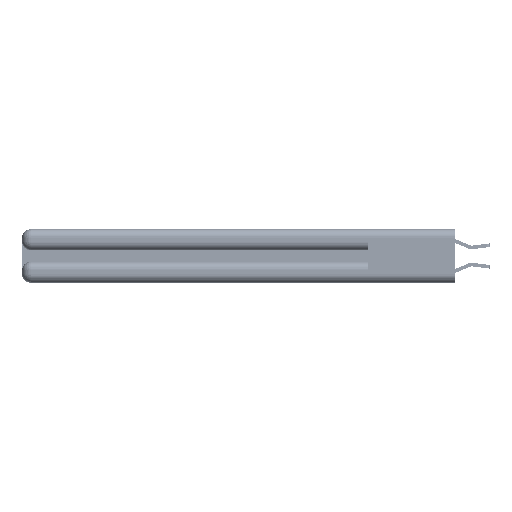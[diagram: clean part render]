
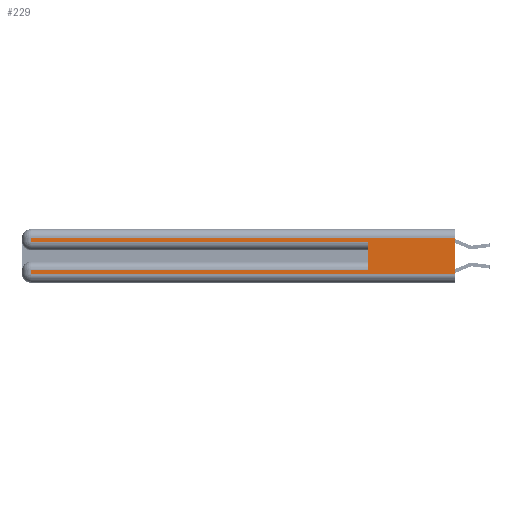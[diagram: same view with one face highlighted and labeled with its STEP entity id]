
A CAD part, left-side view. The second image highlights one B-rep face of the part: STEP entity #229.
In plain terms, the highlighted planar face has unit normal (-1, 0, 0).
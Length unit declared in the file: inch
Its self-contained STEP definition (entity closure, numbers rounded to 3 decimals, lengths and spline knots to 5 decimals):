
#146 = DIRECTION ( 'NONE',  ( 0., 0., -1. ) ) ;
#229 = ADVANCED_FACE ( 'NONE', ( #24275 ), #35878, .F. ) ;
#1392 = CARTESIAN_POINT ( 'NONE',  ( 0., 2.94, 0.31 ) ) ;
#1485 = DIRECTION ( 'NONE',  ( 0., 0., -1. ) ) ;
#1652 = LINE ( 'NONE', #9821, #9694 ) ;
#2906 = DIRECTION ( 'NONE',  ( 0., 0., 1. ) ) ;
#3354 = ORIENTED_EDGE ( 'NONE', *, *, #12501, .T. ) ;
#3734 = LINE ( 'NONE', #18161, #14110 ) ;
#4711 = VERTEX_POINT ( 'NONE', #18787 ) ;
#4900 = VERTEX_POINT ( 'NONE', #19917 ) ;
#5109 = DIRECTION ( 'NONE',  ( 0., 1., 0. ) ) ;
#6617 = VERTEX_POINT ( 'NONE', #23545 ) ;
#6716 = ORIENTED_EDGE ( 'NONE', *, *, #29918, .T. ) ;
#6874 = CARTESIAN_POINT ( 'NONE',  ( 0., 2.94, 0.285 ) ) ;
#9539 = VECTOR ( 'NONE', #30408, 39.37008 ) ;
#9694 = VECTOR ( 'NONE', #26918, 39.37008 ) ;
#9821 = CARTESIAN_POINT ( 'NONE',  ( 0., 0., 0.06 ) ) ;
#9845 = CARTESIAN_POINT ( 'NONE',  ( 0., 0., 0.37 ) ) ;
#9927 = VECTOR ( 'NONE', #5109, 39.37008 ) ;
#10403 = VECTOR ( 'NONE', #15825, 39.37008 ) ;
#11476 = EDGE_LOOP ( 'NONE', ( #21089, #34131, #6716, #29135, #17779, #20069, #21492, #3354 ) ) ;
#11734 = VERTEX_POINT ( 'NONE', #6874 ) ;
#12501 = EDGE_CURVE ( 'NONE', #4900, #4711, #1652, .T. ) ;
#14110 = VECTOR ( 'NONE', #146, 39.37008 ) ;
#14244 = VECTOR ( 'NONE', #37035, 39.37008 ) ;
#15766 = VERTEX_POINT ( 'NONE', #30734 ) ;
#15825 = DIRECTION ( 'NONE',  ( 0., 1., 0. ) ) ;
#16024 = VECTOR ( 'NONE', #2906, 39.37008 ) ;
#16754 = VERTEX_POINT ( 'NONE', #34576 ) ;
#17735 = CARTESIAN_POINT ( 'NONE',  ( 0., 0., 0.285 ) ) ;
#17779 = ORIENTED_EDGE ( 'NONE', *, *, #35022, .F. ) ;
#18161 = CARTESIAN_POINT ( 'NONE',  ( 0., 0., 0.37 ) ) ;
#18787 = CARTESIAN_POINT ( 'NONE',  ( 0., 0., 0.06 ) ) ;
#18814 = CARTESIAN_POINT ( 'NONE',  ( 0., 2.94, 0.37 ) ) ;
#19149 = LINE ( 'NONE', #19717, #9927 ) ;
#19717 = CARTESIAN_POINT ( 'NONE',  ( 0., 0., 0.085 ) ) ;
#19744 = EDGE_CURVE ( 'NONE', #16754, #31587, #21523, .T. ) ;
#19830 = LINE ( 'NONE', #17735, #30695 ) ;
#19917 = CARTESIAN_POINT ( 'NONE',  ( 0., 2.94, 0.06 ) ) ;
#20069 = ORIENTED_EDGE ( 'NONE', *, *, #35955, .T. ) ;
#21089 = ORIENTED_EDGE ( 'NONE', *, *, #23255, .F. ) ;
#21492 = ORIENTED_EDGE ( 'NONE', *, *, #27458, .T. ) ;
#21523 = LINE ( 'NONE', #29721, #10403 ) ;
#22397 = LINE ( 'NONE', #33994, #14244 ) ;
#22463 = CARTESIAN_POINT ( 'NONE',  ( 0., 0.6, 0.145 ) ) ;
#22849 = LINE ( 'NONE', #22463, #16024 ) ;
#23255 = EDGE_CURVE ( 'NONE', #16754, #4711, #3734, .T. ) ;
#23545 = CARTESIAN_POINT ( 'NONE',  ( 0., 2.94, 0.085 ) ) ;
#24275 = FACE_OUTER_BOUND ( 'NONE', #11476, .T. ) ;
#25005 = CARTESIAN_POINT ( 'NONE',  ( 0., 0.6, 0.285 ) ) ;
#26614 = EDGE_CURVE ( 'NONE', #11734, #36471, #19830, .T. ) ;
#26918 = DIRECTION ( 'NONE',  ( 0., -1., 0. ) ) ;
#27318 = DIRECTION ( 'NONE',  ( 1., 0., 0. ) ) ;
#27458 = EDGE_CURVE ( 'NONE', #6617, #4900, #22397, .T. ) ;
#29135 = ORIENTED_EDGE ( 'NONE', *, *, #26614, .T. ) ;
#29721 = CARTESIAN_POINT ( 'NONE',  ( 0., 0., 0.31 ) ) ;
#29918 = EDGE_CURVE ( 'NONE', #31587, #11734, #30597, .T. ) ;
#30408 = DIRECTION ( 'NONE',  ( 0., 0., -1. ) ) ;
#30597 = LINE ( 'NONE', #18814, #9539 ) ;
#30695 = VECTOR ( 'NONE', #32000, 39.37008 ) ;
#30734 = CARTESIAN_POINT ( 'NONE',  ( 0., 0.6, 0.085 ) ) ;
#31587 = VERTEX_POINT ( 'NONE', #1392 ) ;
#32000 = DIRECTION ( 'NONE',  ( 0., -1., 0. ) ) ;
#33994 = CARTESIAN_POINT ( 'NONE',  ( 0., 2.94, 0.37 ) ) ;
#34131 = ORIENTED_EDGE ( 'NONE', *, *, #19744, .T. ) ;
#34576 = CARTESIAN_POINT ( 'NONE',  ( 0., 0., 0.31 ) ) ;
#35022 = EDGE_CURVE ( 'NONE', #15766, #36471, #22849, .T. ) ;
#35192 = AXIS2_PLACEMENT_3D ( 'NONE', #9845, #27318, #1485 ) ;
#35878 = PLANE ( 'NONE',  #35192 ) ;
#35955 = EDGE_CURVE ( 'NONE', #15766, #6617, #19149, .T. ) ;
#36471 = VERTEX_POINT ( 'NONE', #25005 ) ;
#37035 = DIRECTION ( 'NONE',  ( 0., 0., -1. ) ) ;
